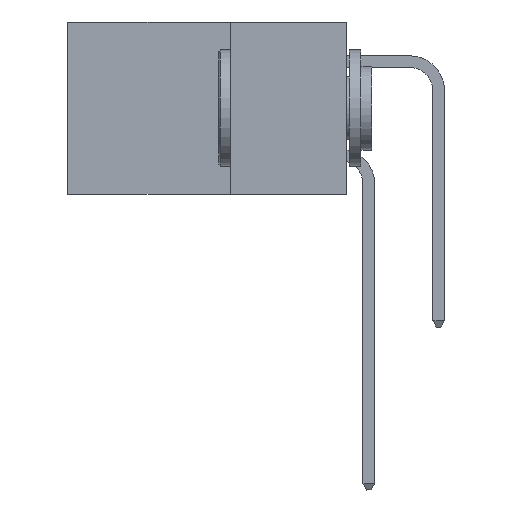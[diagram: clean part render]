
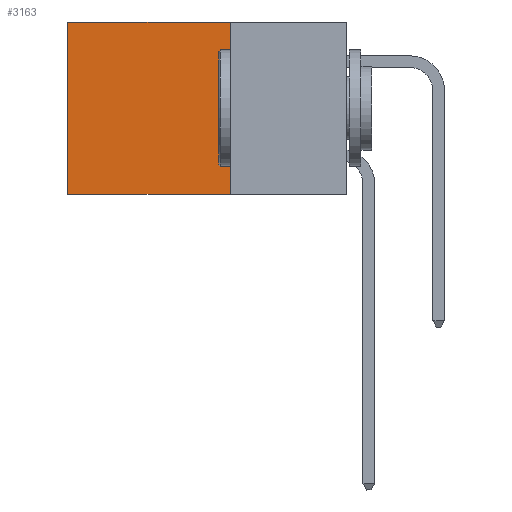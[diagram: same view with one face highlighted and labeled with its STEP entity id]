
A CAD part, left-side view. The second image highlights one B-rep face of the part: STEP entity #3163.
In plain terms, the highlighted planar face has unit normal (-1, 0, 0).
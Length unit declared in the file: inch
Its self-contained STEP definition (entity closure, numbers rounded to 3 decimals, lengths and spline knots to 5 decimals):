
#3127 = FACE_OUTER_BOUND ( 'NONE', #22589, .T. ) ;
#3163 = ADVANCED_FACE ( 'NONE', ( #3127 ), #22033, .F. ) ;
#3275 = EDGE_CURVE ( 'NONE', #3981, #24302, #10879, .T. ) ;
#3561 = CARTESIAN_POINT ( 'NONE',  ( 0.2875, 0.25, 0. ) ) ;
#3981 = VERTEX_POINT ( 'NONE', #15968 ) ;
#4721 = VECTOR ( 'NONE', #22473, 39.37008 ) ;
#5555 = CARTESIAN_POINT ( 'NONE',  ( 0.2875, 0.25, 0. ) ) ;
#5759 = VERTEX_POINT ( 'NONE', #19109 ) ;
#6802 = LINE ( 'NONE', #21044, #24603 ) ;
#7845 = LINE ( 'NONE', #3561, #24976 ) ;
#9053 = LINE ( 'NONE', #5555, #13584 ) ;
#10879 = LINE ( 'NONE', #18422, #4721 ) ;
#11398 = DIRECTION ( 'NONE',  ( 1., 0., 0. ) ) ;
#11563 = EDGE_CURVE ( 'NONE', #13093, #24302, #6802, .T. ) ;
#11751 = CARTESIAN_POINT ( 'NONE',  ( 0.2875, 0.6, -0.37 ) ) ;
#13093 = VERTEX_POINT ( 'NONE', #21443 ) ;
#13584 = VECTOR ( 'NONE', #22110, 39.37008 ) ;
#14784 = ORIENTED_EDGE ( 'NONE', *, *, #11563, .T. ) ;
#15968 = CARTESIAN_POINT ( 'NONE',  ( 0.2875, 0.25, -0.37 ) ) ;
#18184 = AXIS2_PLACEMENT_3D ( 'NONE', #22125, #11398, #19714 ) ;
#18422 = CARTESIAN_POINT ( 'NONE',  ( 0.2875, 0.25, -0.37 ) ) ;
#19109 = CARTESIAN_POINT ( 'NONE',  ( 0.2875, 0.25, 0. ) ) ;
#19235 = EDGE_CURVE ( 'NONE', #5759, #13093, #7845, .T. ) ;
#19714 = DIRECTION ( 'NONE',  ( 0., 0., -1. ) ) ;
#19936 = DIRECTION ( 'NONE',  ( 0., 0., -1. ) ) ;
#20245 = ORIENTED_EDGE ( 'NONE', *, *, #3275, .F. ) ;
#20710 = EDGE_CURVE ( 'NONE', #5759, #3981, #9053, .T. ) ;
#21044 = CARTESIAN_POINT ( 'NONE',  ( 0.2875, 0.6, 0. ) ) ;
#21279 = ORIENTED_EDGE ( 'NONE', *, *, #20710, .F. ) ;
#21443 = CARTESIAN_POINT ( 'NONE',  ( 0.2875, 0.6, 0. ) ) ;
#22033 = PLANE ( 'NONE',  #18184 ) ;
#22110 = DIRECTION ( 'NONE',  ( 0., 0., -1. ) ) ;
#22125 = CARTESIAN_POINT ( 'NONE',  ( 0.2875, 0.25, 0. ) ) ;
#22298 = ORIENTED_EDGE ( 'NONE', *, *, #19235, .T. ) ;
#22473 = DIRECTION ( 'NONE',  ( 0., 1., 0. ) ) ;
#22589 = EDGE_LOOP ( 'NONE', ( #14784, #20245, #21279, #22298 ) ) ;
#24015 = DIRECTION ( 'NONE',  ( 0., 1., 0. ) ) ;
#24302 = VERTEX_POINT ( 'NONE', #11751 ) ;
#24603 = VECTOR ( 'NONE', #19936, 39.37008 ) ;
#24976 = VECTOR ( 'NONE', #24015, 39.37008 ) ;
